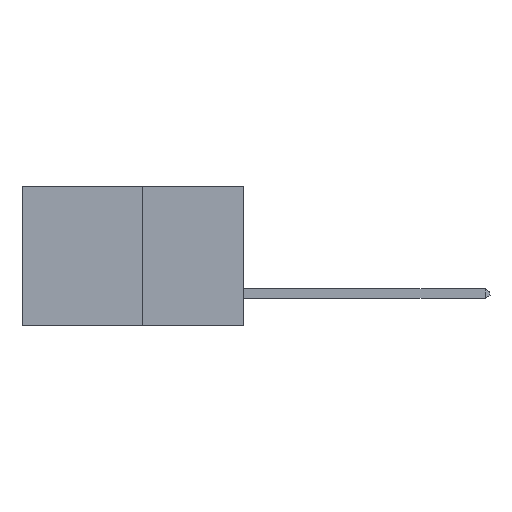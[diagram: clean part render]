
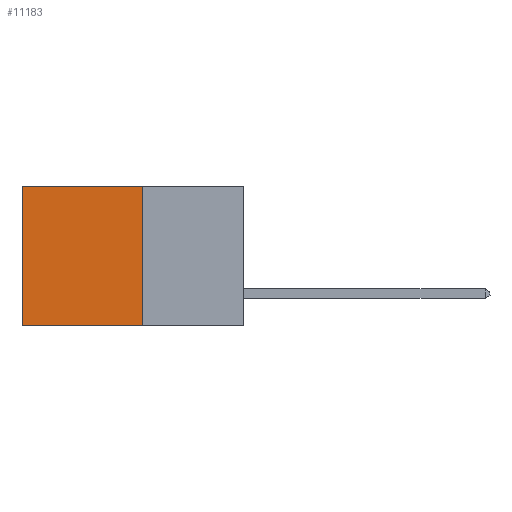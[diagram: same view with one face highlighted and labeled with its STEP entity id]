
A CAD part, left-side view. The second image highlights one B-rep face of the part: STEP entity #11183.
In plain terms, the highlighted planar face has unit normal (-1, 0, 0).
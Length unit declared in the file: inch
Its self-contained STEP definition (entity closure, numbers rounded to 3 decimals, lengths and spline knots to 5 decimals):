
#356 = DIRECTION ( 'NONE',  ( 0., 0., -1. ) ) ;
#992 = ORIENTED_EDGE ( 'NONE', *, *, #11663, .F. ) ;
#1072 = ORIENTED_EDGE ( 'NONE', *, *, #4469, .T. ) ;
#1263 = PLANE ( 'NONE',  #11327 ) ;
#1425 = EDGE_CURVE ( 'NONE', #7555, #6608, #2486, .T. ) ;
#2457 = DIRECTION ( 'NONE',  ( 1., 0., 0. ) ) ;
#2486 = LINE ( 'NONE', #6314, #2855 ) ;
#2855 = VECTOR ( 'NONE', #12197, 39.37008 ) ;
#3339 = LINE ( 'NONE', #13762, #9082 ) ;
#3546 = ORIENTED_EDGE ( 'NONE', *, *, #14191, .F. ) ;
#4469 = EDGE_CURVE ( 'NONE', #13667, #7555, #12528, .T. ) ;
#4950 = CARTESIAN_POINT ( 'NONE',  ( 0.277, 0.27, 0. ) ) ;
#5837 = LINE ( 'NONE', #13987, #14361 ) ;
#6293 = ORIENTED_EDGE ( 'NONE', *, *, #1425, .T. ) ;
#6314 = CARTESIAN_POINT ( 'NONE',  ( 0.277, 0.59, -0.37 ) ) ;
#6566 = VECTOR ( 'NONE', #13835, 39.37008 ) ;
#6608 = VERTEX_POINT ( 'NONE', #10925 ) ;
#6617 = CARTESIAN_POINT ( 'NONE',  ( 0.277, 0.27, -0.37 ) ) ;
#7555 = VERTEX_POINT ( 'NONE', #11366 ) ;
#9082 = VECTOR ( 'NONE', #12686, 39.37008 ) ;
#9339 = CARTESIAN_POINT ( 'NONE',  ( 0.277, 0.27, -0.37 ) ) ;
#10475 = DIRECTION ( 'NONE',  ( 0., 0., -1. ) ) ;
#10925 = CARTESIAN_POINT ( 'NONE',  ( 0.277, 0.59, -0.37 ) ) ;
#11183 = ADVANCED_FACE ( 'NONE', ( #13232 ), #1263, .F. ) ;
#11327 = AXIS2_PLACEMENT_3D ( 'NONE', #9339, #2457, #10475 ) ;
#11366 = CARTESIAN_POINT ( 'NONE',  ( 0.277, 0.59, 0. ) ) ;
#11653 = CARTESIAN_POINT ( 'NONE',  ( 0.277, 0.27, 0. ) ) ;
#11663 = EDGE_CURVE ( 'NONE', #13350, #6608, #3339, .T. ) ;
#12197 = DIRECTION ( 'NONE',  ( 0., 0., -1. ) ) ;
#12322 = EDGE_LOOP ( 'NONE', ( #6293, #992, #3546, #1072 ) ) ;
#12528 = LINE ( 'NONE', #11653, #6566 ) ;
#12686 = DIRECTION ( 'NONE',  ( 0., 1., 0. ) ) ;
#13232 = FACE_OUTER_BOUND ( 'NONE', #12322, .T. ) ;
#13350 = VERTEX_POINT ( 'NONE', #6617 ) ;
#13667 = VERTEX_POINT ( 'NONE', #4950 ) ;
#13762 = CARTESIAN_POINT ( 'NONE',  ( 0.277, 0.27, -0.37 ) ) ;
#13835 = DIRECTION ( 'NONE',  ( 0., 1., 0. ) ) ;
#13987 = CARTESIAN_POINT ( 'NONE',  ( 0.277, 0.27, -0.37 ) ) ;
#14191 = EDGE_CURVE ( 'NONE', #13667, #13350, #5837, .T. ) ;
#14361 = VECTOR ( 'NONE', #356, 39.37008 ) ;
